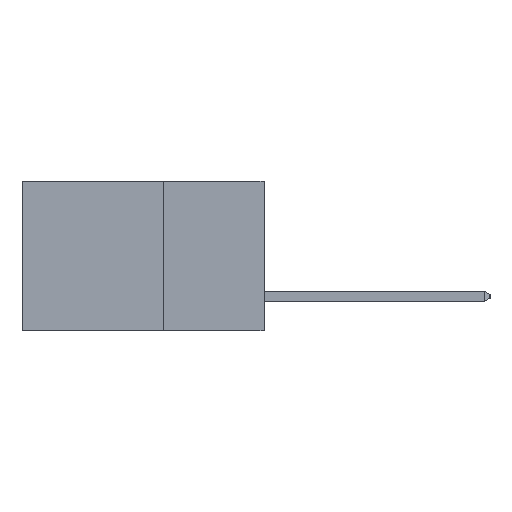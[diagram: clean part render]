
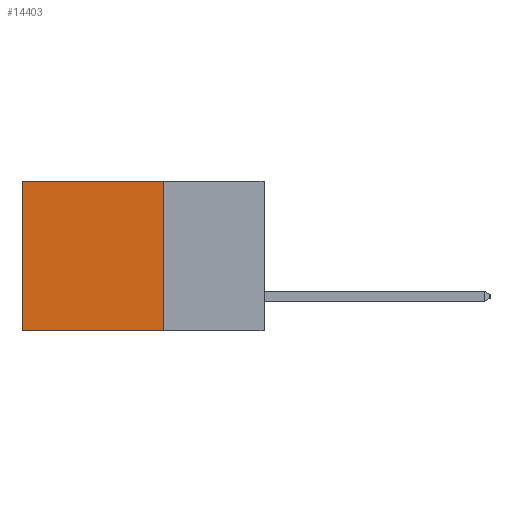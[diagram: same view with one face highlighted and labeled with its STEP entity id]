
A CAD part, left-side view. The second image highlights one B-rep face of the part: STEP entity #14403.
In plain terms, the highlighted planar face has unit normal (-1, 0, 0).
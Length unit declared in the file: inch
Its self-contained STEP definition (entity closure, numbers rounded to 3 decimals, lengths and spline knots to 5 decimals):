
#991 = DIRECTION ( 'NONE',  ( 1., 0., 0. ) ) ;
#2584 = VERTEX_POINT ( 'NONE', #6255 ) ;
#2664 = EDGE_CURVE ( 'NONE', #13988, #2584, #18194, .T. ) ;
#2859 = CARTESIAN_POINT ( 'NONE',  ( 0.2615, 0.25, -0.37 ) ) ;
#2924 = EDGE_LOOP ( 'NONE', ( #8237, #23597, #5864, #3943 ) ) ;
#3943 = ORIENTED_EDGE ( 'NONE', *, *, #2664, .T. ) ;
#4198 = DIRECTION ( 'NONE',  ( 0., 1., 0. ) ) ;
#4803 = EDGE_CURVE ( 'NONE', #2584, #9832, #8502, .T. ) ;
#4841 = DIRECTION ( 'NONE',  ( 0., 1., 0. ) ) ;
#4884 = CARTESIAN_POINT ( 'NONE',  ( 0.2615, 0.25, 0. ) ) ;
#5412 = CARTESIAN_POINT ( 'NONE',  ( 0.2615, 0.6, -0.37 ) ) ;
#5647 = DIRECTION ( 'NONE',  ( 0., 0., -1. ) ) ;
#5864 = ORIENTED_EDGE ( 'NONE', *, *, #25348, .F. ) ;
#6109 = LINE ( 'NONE', #12090, #10792 ) ;
#6255 = CARTESIAN_POINT ( 'NONE',  ( 0.2615, 0.6, 0. ) ) ;
#6826 = VERTEX_POINT ( 'NONE', #18682 ) ;
#7677 = VECTOR ( 'NONE', #4841, 39.37008 ) ;
#8237 = ORIENTED_EDGE ( 'NONE', *, *, #4803, .T. ) ;
#8502 = LINE ( 'NONE', #5412, #13789 ) ;
#9832 = VERTEX_POINT ( 'NONE', #23171 ) ;
#10509 = VECTOR ( 'NONE', #4198, 39.37008 ) ;
#10792 = VECTOR ( 'NONE', #23807, 39.37008 ) ;
#12090 = CARTESIAN_POINT ( 'NONE',  ( 0.2615, 0.25, -0.37 ) ) ;
#13230 = CARTESIAN_POINT ( 'NONE',  ( 0.2615, 0.25, 0. ) ) ;
#13601 = EDGE_CURVE ( 'NONE', #6826, #9832, #20947, .T. ) ;
#13789 = VECTOR ( 'NONE', #5647, 39.37008 ) ;
#13988 = VERTEX_POINT ( 'NONE', #13230 ) ;
#14263 = FACE_OUTER_BOUND ( 'NONE', #2924, .T. ) ;
#14403 = ADVANCED_FACE ( 'NONE', ( #14263 ), #20628, .F. ) ;
#14855 = DIRECTION ( 'NONE',  ( 0., 0., -1. ) ) ;
#16239 = AXIS2_PLACEMENT_3D ( 'NONE', #2859, #991, #14855 ) ;
#18194 = LINE ( 'NONE', #4884, #7677 ) ;
#18682 = CARTESIAN_POINT ( 'NONE',  ( 0.2615, 0.25, -0.37 ) ) ;
#20628 = PLANE ( 'NONE',  #16239 ) ;
#20947 = LINE ( 'NONE', #23824, #10509 ) ;
#23171 = CARTESIAN_POINT ( 'NONE',  ( 0.2615, 0.6, -0.37 ) ) ;
#23597 = ORIENTED_EDGE ( 'NONE', *, *, #13601, .F. ) ;
#23807 = DIRECTION ( 'NONE',  ( 0., 0., -1. ) ) ;
#23824 = CARTESIAN_POINT ( 'NONE',  ( 0.2615, 0.25, -0.37 ) ) ;
#25348 = EDGE_CURVE ( 'NONE', #13988, #6826, #6109, .T. ) ;
